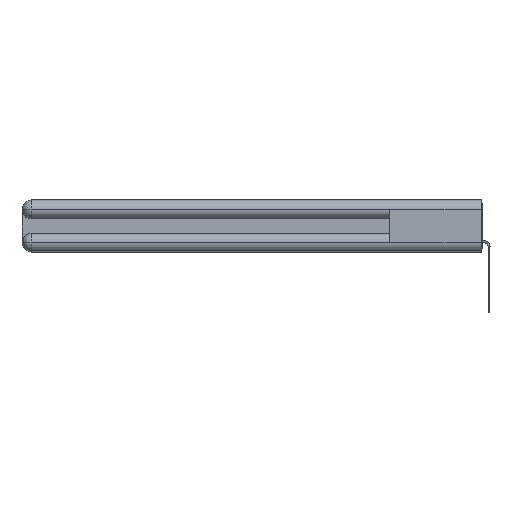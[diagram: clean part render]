
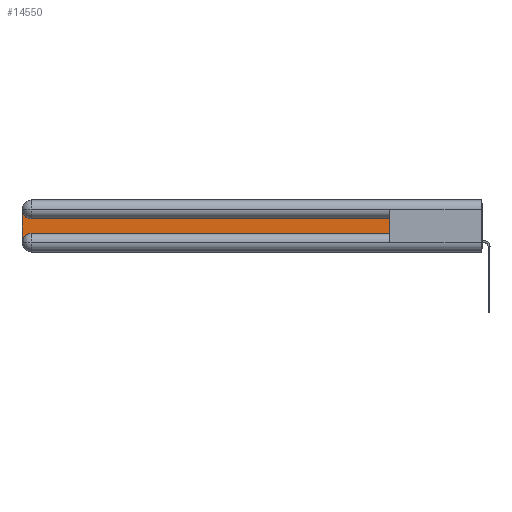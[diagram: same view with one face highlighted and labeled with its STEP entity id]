
A CAD part, left-side view. The second image highlights one B-rep face of the part: STEP entity #14550.
In plain terms, the highlighted planar face has unit normal (-1, 0, 0).
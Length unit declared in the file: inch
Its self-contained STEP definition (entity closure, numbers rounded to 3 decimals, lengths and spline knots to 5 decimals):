
#240 = FACE_OUTER_BOUND ( 'NONE', #10022, .T. ) ;
#378 = CARTESIAN_POINT ( 'NONE',  ( 0.075, 3., -0.1225 ) ) ;
#525 = DIRECTION ( 'NONE',  ( 1., 0., 0. ) ) ;
#840 = ORIENTED_EDGE ( 'NONE', *, *, #24201, .T. ) ;
#953 = AXIS2_PLACEMENT_3D ( 'NONE', #24146, #10617, #23594 ) ;
#1987 = ORIENTED_EDGE ( 'NONE', *, *, #7107, .T. ) ;
#2454 = LINE ( 'NONE', #23938, #18003 ) ;
#2736 = CARTESIAN_POINT ( 'NONE',  ( 0.075, 2.94, -0.0625 ) ) ;
#2779 = VECTOR ( 'NONE', #27279, 39.37008 ) ;
#3220 = CARTESIAN_POINT ( 'NONE',  ( 0.075, 3., -0.2175 ) ) ;
#3720 = AXIS2_PLACEMENT_3D ( 'NONE', #2736, #11555, #6916 ) ;
#4877 = CARTESIAN_POINT ( 'NONE',  ( 0.075, 0.6, -0.1225 ) ) ;
#5003 = ORIENTED_EDGE ( 'NONE', *, *, #24233, .T. ) ;
#5510 = AXIS2_PLACEMENT_3D ( 'NONE', #378, #525, #13813 ) ;
#5884 = VERTEX_POINT ( 'NONE', #14900 ) ;
#5932 = VERTEX_POINT ( 'NONE', #10863 ) ;
#6052 = CARTESIAN_POINT ( 'NONE',  ( 0.075, 3., -0.0625 ) ) ;
#6315 = VERTEX_POINT ( 'NONE', #6052 ) ;
#6916 = DIRECTION ( 'NONE',  ( 0., 0., -1. ) ) ;
#7107 = EDGE_CURVE ( 'NONE', #13641, #11485, #22858, .T. ) ;
#7148 = CARTESIAN_POINT ( 'NONE',  ( 0.075, 2.94, -0.2175 ) ) ;
#10022 = EDGE_LOOP ( 'NONE', ( #24735, #14875, #5003, #27378, #840, #1987 ) ) ;
#10293 = LINE ( 'NONE', #16899, #11567 ) ;
#10315 = VECTOR ( 'NONE', #20544, 39.37008 ) ;
#10442 = LINE ( 'NONE', #3220, #2779 ) ;
#10617 = DIRECTION ( 'NONE',  ( 1., 0., 0. ) ) ;
#10863 = CARTESIAN_POINT ( 'NONE',  ( 0.075, 2.94, -0.1225 ) ) ;
#11485 = VERTEX_POINT ( 'NONE', #4877 ) ;
#11555 = DIRECTION ( 'NONE',  ( 1., 0., 0. ) ) ;
#11567 = VECTOR ( 'NONE', #19059, 39.37008 ) ;
#11570 = CIRCLE ( 'NONE', #3720, 0.06 ) ;
#13641 = VERTEX_POINT ( 'NONE', #22838 ) ;
#13813 = DIRECTION ( 'NONE',  ( 0., 0., -1. ) ) ;
#14550 = ADVANCED_FACE ( 'NONE', ( #240 ), #17844, .F. ) ;
#14875 = ORIENTED_EDGE ( 'NONE', *, *, #22814, .T. ) ;
#14900 = CARTESIAN_POINT ( 'NONE',  ( 0.075, 3., -0.2775 ) ) ;
#16899 = CARTESIAN_POINT ( 'NONE',  ( 0.075, 0.6, -0.2175 ) ) ;
#17442 = EDGE_CURVE ( 'NONE', #5884, #28274, #27634, .T. ) ;
#17844 = PLANE ( 'NONE',  #5510 ) ;
#17849 = EDGE_CURVE ( 'NONE', #11485, #5932, #2454, .T. ) ;
#18003 = VECTOR ( 'NONE', #24083, 39.37008 ) ;
#19059 = DIRECTION ( 'NONE',  ( 0., -1., 0. ) ) ;
#20544 = DIRECTION ( 'NONE',  ( 0., 0., 1. ) ) ;
#22814 = EDGE_CURVE ( 'NONE', #5932, #6315, #11570, .T. ) ;
#22838 = CARTESIAN_POINT ( 'NONE',  ( 0.075, 0.6, -0.2175 ) ) ;
#22858 = LINE ( 'NONE', #26867, #10315 ) ;
#23594 = DIRECTION ( 'NONE',  ( 0., 0., -1. ) ) ;
#23938 = CARTESIAN_POINT ( 'NONE',  ( 0.075, 0.6, -0.1225 ) ) ;
#24083 = DIRECTION ( 'NONE',  ( 0., 1., 0. ) ) ;
#24146 = CARTESIAN_POINT ( 'NONE',  ( 0.075, 2.94, -0.2775 ) ) ;
#24201 = EDGE_CURVE ( 'NONE', #28274, #13641, #10293, .T. ) ;
#24233 = EDGE_CURVE ( 'NONE', #6315, #5884, #10442, .T. ) ;
#24735 = ORIENTED_EDGE ( 'NONE', *, *, #17849, .T. ) ;
#26867 = CARTESIAN_POINT ( 'NONE',  ( 0.075, 0.6, -0.2175 ) ) ;
#27279 = DIRECTION ( 'NONE',  ( 0., 0., -1. ) ) ;
#27378 = ORIENTED_EDGE ( 'NONE', *, *, #17442, .T. ) ;
#27634 = CIRCLE ( 'NONE', #953, 0.06 ) ;
#28274 = VERTEX_POINT ( 'NONE', #7148 ) ;
